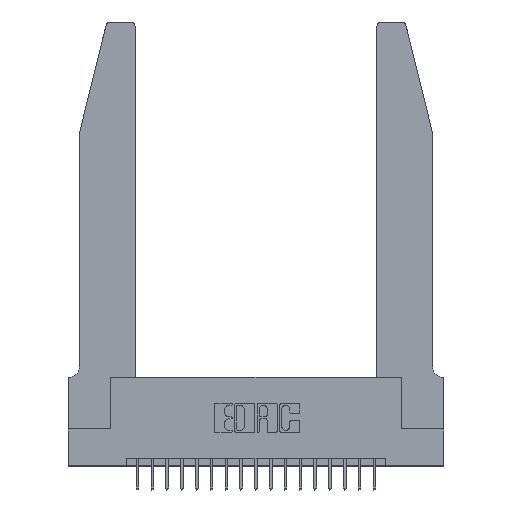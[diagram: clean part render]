
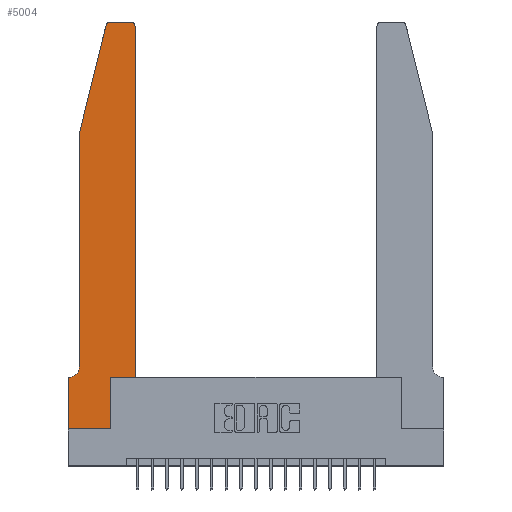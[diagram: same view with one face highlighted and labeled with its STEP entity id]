
A CAD part, top view. The second image highlights one B-rep face of the part: STEP entity #5004.
In plain terms, the highlighted planar face has unit normal (0, 0, 1).
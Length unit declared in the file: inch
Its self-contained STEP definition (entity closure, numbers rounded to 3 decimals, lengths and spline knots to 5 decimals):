
#316 = VERTEX_POINT ( 'NONE', #7975 ) ;
#624 = CARTESIAN_POINT ( 'NONE',  ( 0.0755, 0.35, 0.37 ) ) ;
#990 = DIRECTION ( 'NONE',  ( 1., 0., 0. ) ) ;
#1227 = VECTOR ( 'NONE', #5634, 39.37008 ) ;
#1559 = VERTEX_POINT ( 'NONE', #21024 ) ;
#1569 = LINE ( 'NONE', #5032, #5598 ) ;
#1591 = CIRCLE ( 'NONE', #20777, 0.07 ) ;
#1840 = VERTEX_POINT ( 'NONE', #11845 ) ;
#1859 = DIRECTION ( 'NONE',  ( 1., 0., 0. ) ) ;
#1943 = EDGE_CURVE ( 'NONE', #9316, #1559, #7477, .T. ) ;
#2251 = CARTESIAN_POINT ( 'NONE',  ( 0., 0.35, 0.37 ) ) ;
#2355 = VERTEX_POINT ( 'NONE', #19152 ) ;
#2561 = ORIENTED_EDGE ( 'NONE', *, *, #10657, .T. ) ;
#2575 = VERTEX_POINT ( 'NONE', #11493 ) ;
#2719 = CARTESIAN_POINT ( 'NONE',  ( 0.4205, 2.72, 0.37 ) ) ;
#2726 = EDGE_CURVE ( 'NONE', #8242, #2355, #1591, .T. ) ;
#2758 = LINE ( 'NONE', #19487, #19774 ) ;
#3077 = CARTESIAN_POINT ( 'NONE',  ( 0.4505, 0.35, 0.37 ) ) ;
#3081 = VECTOR ( 'NONE', #8129, 39.37008 ) ;
#3551 = ORIENTED_EDGE ( 'NONE', *, *, #20086, .T. ) ;
#3721 = EDGE_CURVE ( 'NONE', #18763, #15145, #5301, .T. ) ;
#3878 = VERTEX_POINT ( 'NONE', #8713 ) ;
#4399 = DIRECTION ( 'NONE',  ( 1., 0., 0. ) ) ;
#4670 = ORIENTED_EDGE ( 'NONE', *, *, #11629, .T. ) ;
#4923 = DIRECTION ( 'NONE',  ( 0., 0., 1. ) ) ;
#4987 = DIRECTION ( 'NONE',  ( -1., 0., 0. ) ) ;
#5004 = ADVANCED_FACE ( 'NONE', ( #13040 ), #13910, .T. ) ;
#5032 = CARTESIAN_POINT ( 'NONE',  ( 0.0755, 2., 0.37 ) ) ;
#5301 = LINE ( 'NONE', #19520, #17924 ) ;
#5455 = VECTOR ( 'NONE', #1859, 39.37008 ) ;
#5598 = VECTOR ( 'NONE', #13353, 39.37008 ) ;
#5634 = DIRECTION ( 'NONE',  ( 0., -1., 0. ) ) ;
#6265 = ORIENTED_EDGE ( 'NONE', *, *, #3721, .T. ) ;
#6497 = DIRECTION ( 'NONE',  ( 0., -1., 0. ) ) ;
#6578 = AXIS2_PLACEMENT_3D ( 'NONE', #2251, #20414, #10659 ) ;
#6672 = LINE ( 'NONE', #9447, #10523 ) ;
#6735 = LINE ( 'NONE', #624, #19281 ) ;
#6769 = VERTEX_POINT ( 'NONE', #14989 ) ;
#6972 = DIRECTION ( 'NONE',  ( 0., 0., -1. ) ) ;
#7218 = EDGE_CURVE ( 'NONE', #6769, #9316, #18572, .T. ) ;
#7477 = CIRCLE ( 'NONE', #17248, 0.03 ) ;
#7535 = LINE ( 'NONE', #3077, #3081 ) ;
#7601 = ORIENTED_EDGE ( 'NONE', *, *, #10240, .T. ) ;
#7975 = CARTESIAN_POINT ( 'NONE',  ( 0.4505, 2.72, 0.37 ) ) ;
#8020 = EDGE_LOOP ( 'NONE', ( #16718, #15351, #3551, #16431, #11101, #7601, #6265, #4670, #2561, #8922, #19412, #9361 ) ) ;
#8129 = DIRECTION ( 'NONE',  ( 0., 1., 0. ) ) ;
#8242 = VERTEX_POINT ( 'NONE', #21527 ) ;
#8713 = CARTESIAN_POINT ( 'NONE',  ( 0.4505, 0.35, 0.37 ) ) ;
#8922 = ORIENTED_EDGE ( 'NONE', *, *, #16437, .T. ) ;
#9316 = VERTEX_POINT ( 'NONE', #12745 ) ;
#9361 = ORIENTED_EDGE ( 'NONE', *, *, #9783, .T. ) ;
#9447 = CARTESIAN_POINT ( 'NONE',  ( 0., 0., 0.37 ) ) ;
#9705 = LINE ( 'NONE', #15502, #1227 ) ;
#9783 = EDGE_CURVE ( 'NONE', #316, #6769, #21469, .T. ) ;
#9908 = DIRECTION ( 'NONE',  ( 0., 1., 0. ) ) ;
#10240 = EDGE_CURVE ( 'NONE', #2355, #18763, #6735, .T. ) ;
#10523 = VECTOR ( 'NONE', #990, 39.37008 ) ;
#10657 = EDGE_CURVE ( 'NONE', #16674, #1840, #2758, .T. ) ;
#10659 = DIRECTION ( 'NONE',  ( 1., 0., 0. ) ) ;
#11101 = ORIENTED_EDGE ( 'NONE', *, *, #2726, .T. ) ;
#11493 = CARTESIAN_POINT ( 'NONE',  ( 0.0755, 2., 0.37 ) ) ;
#11585 = CARTESIAN_POINT ( 'NONE',  ( 0.2605, 2.75, 0.37 ) ) ;
#11629 = EDGE_CURVE ( 'NONE', #15145, #16674, #6672, .T. ) ;
#11845 = CARTESIAN_POINT ( 'NONE',  ( 0.2865, 0.35, 0.37 ) ) ;
#12743 = AXIS2_PLACEMENT_3D ( 'NONE', #2719, #14328, #4399 ) ;
#12745 = CARTESIAN_POINT ( 'NONE',  ( 0.284, 2.75, 0.37 ) ) ;
#12780 = EDGE_CURVE ( 'NONE', #2575, #8242, #9705, .T. ) ;
#13040 = FACE_OUTER_BOUND ( 'NONE', #8020, .T. ) ;
#13217 = LINE ( 'NONE', #13519, #5455 ) ;
#13353 = DIRECTION ( 'NONE',  ( -0.239, -0.971, 0. ) ) ;
#13519 = CARTESIAN_POINT ( 'NONE',  ( 0.4505, 0.35, 0.37 ) ) ;
#13726 = CARTESIAN_POINT ( 'NONE',  ( 0., 0., 0.37 ) ) ;
#13910 = PLANE ( 'NONE',  #6578 ) ;
#14328 = DIRECTION ( 'NONE',  ( 0., 0., 1. ) ) ;
#14844 = CARTESIAN_POINT ( 'NONE',  ( 0.284, 2.72, 0.37 ) ) ;
#14989 = CARTESIAN_POINT ( 'NONE',  ( 0.4205, 2.75, 0.37 ) ) ;
#15145 = VERTEX_POINT ( 'NONE', #13726 ) ;
#15351 = ORIENTED_EDGE ( 'NONE', *, *, #1943, .T. ) ;
#15502 = CARTESIAN_POINT ( 'NONE',  ( 0.0755, 2., 0.37 ) ) ;
#16431 = ORIENTED_EDGE ( 'NONE', *, *, #12780, .T. ) ;
#16437 = EDGE_CURVE ( 'NONE', #1840, #3878, #13217, .T. ) ;
#16478 = DIRECTION ( 'NONE',  ( 1., 0., 0. ) ) ;
#16540 = VECTOR ( 'NONE', #4987, 39.37008 ) ;
#16674 = VERTEX_POINT ( 'NONE', #17441 ) ;
#16718 = ORIENTED_EDGE ( 'NONE', *, *, #7218, .T. ) ;
#16772 = EDGE_CURVE ( 'NONE', #3878, #316, #7535, .T. ) ;
#16794 = CARTESIAN_POINT ( 'NONE',  ( 0.0055, 0.42, 0.37 ) ) ;
#17248 = AXIS2_PLACEMENT_3D ( 'NONE', #14844, #4923, #16478 ) ;
#17441 = CARTESIAN_POINT ( 'NONE',  ( 0.2865, 0., 0.37 ) ) ;
#17924 = VECTOR ( 'NONE', #6497, 39.37008 ) ;
#18431 = DIRECTION ( 'NONE',  ( -1., 0., 0. ) ) ;
#18497 = CARTESIAN_POINT ( 'NONE',  ( 0., 0.35, 0.37 ) ) ;
#18572 = LINE ( 'NONE', #11585, #16540 ) ;
#18763 = VERTEX_POINT ( 'NONE', #18497 ) ;
#18925 = DIRECTION ( 'NONE',  ( -1., 0., 0. ) ) ;
#19152 = CARTESIAN_POINT ( 'NONE',  ( 0.0055, 0.35, 0.37 ) ) ;
#19281 = VECTOR ( 'NONE', #18925, 39.37008 ) ;
#19412 = ORIENTED_EDGE ( 'NONE', *, *, #16772, .T. ) ;
#19487 = CARTESIAN_POINT ( 'NONE',  ( 0.2865, 0.35, 0.37 ) ) ;
#19520 = CARTESIAN_POINT ( 'NONE',  ( 0., 0., 0.37 ) ) ;
#19774 = VECTOR ( 'NONE', #9908, 39.37008 ) ;
#20086 = EDGE_CURVE ( 'NONE', #1559, #2575, #1569, .T. ) ;
#20414 = DIRECTION ( 'NONE',  ( 0., 0., 1. ) ) ;
#20777 = AXIS2_PLACEMENT_3D ( 'NONE', #16794, #6972, #18431 ) ;
#21024 = CARTESIAN_POINT ( 'NONE',  ( 0.25487, 2.72718, 0.37 ) ) ;
#21469 = CIRCLE ( 'NONE', #12743, 0.03 ) ;
#21527 = CARTESIAN_POINT ( 'NONE',  ( 0.0755, 0.42, 0.37 ) ) ;
